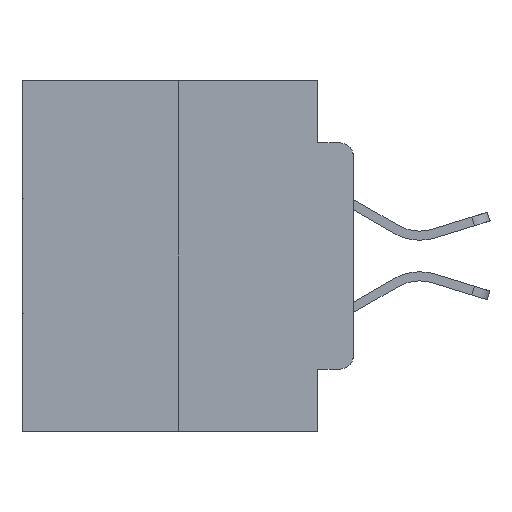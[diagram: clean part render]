
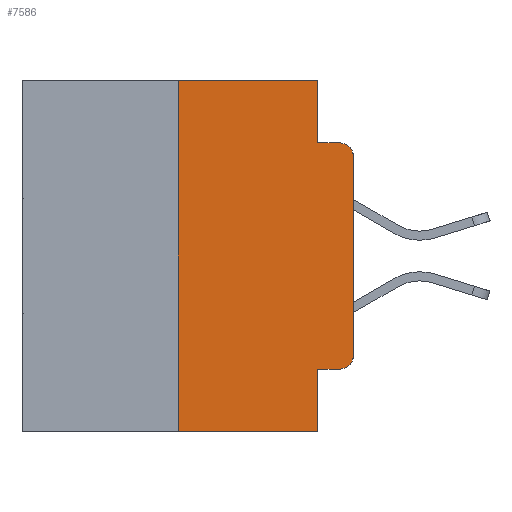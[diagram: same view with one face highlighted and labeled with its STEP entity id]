
A CAD part, left-side view. The second image highlights one B-rep face of the part: STEP entity #7586.
In plain terms, the highlighted planar face has unit normal (-1, 0, 0).
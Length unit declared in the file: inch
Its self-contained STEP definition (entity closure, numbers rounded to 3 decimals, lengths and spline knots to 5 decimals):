
#863 = ORIENTED_EDGE ( 'NONE', *, *, #16979, .F. ) ;
#1055 = CARTESIAN_POINT ( 'NONE',  ( 0., 0.25, -0.5 ) ) ;
#2234 = CIRCLE ( 'NONE', #12386, 0.02 ) ;
#2438 = ORIENTED_EDGE ( 'NONE', *, *, #23348, .F. ) ;
#4496 = CARTESIAN_POINT ( 'NONE',  ( 0., 0.051, 0. ) ) ;
#4684 = CARTESIAN_POINT ( 'NONE',  ( 0., 0., 0. ) ) ;
#5418 = VERTEX_POINT ( 'NONE', #18519 ) ;
#5578 = DIRECTION ( 'NONE',  ( 0., 0., -1. ) ) ;
#5652 = VECTOR ( 'NONE', #28266, 39.37008 ) ;
#5811 = VERTEX_POINT ( 'NONE', #4496 ) ;
#6142 = PLANE ( 'NONE',  #23346 ) ;
#6863 = LINE ( 'NONE', #19147, #18099 ) ;
#7013 = DIRECTION ( 'NONE',  ( 0., 0., 1. ) ) ;
#7075 = VECTOR ( 'NONE', #21052, 39.37008 ) ;
#7295 = LINE ( 'NONE', #7904, #19167 ) ;
#7436 = VERTEX_POINT ( 'NONE', #27648 ) ;
#7541 = LINE ( 'NONE', #4684, #18737 ) ;
#7586 = ADVANCED_FACE ( 'NONE', ( #21837 ), #6142, .F. ) ;
#7904 = CARTESIAN_POINT ( 'NONE',  ( 0., 0.051, 0. ) ) ;
#8372 = EDGE_CURVE ( 'NONE', #18516, #13982, #7541, .T. ) ;
#8602 = LINE ( 'NONE', #24713, #13903 ) ;
#8946 = CARTESIAN_POINT ( 'NONE',  ( 0., 0.051, -0.0885 ) ) ;
#9190 = EDGE_CURVE ( 'NONE', #9930, #7436, #15619, .T. ) ;
#9440 = ORIENTED_EDGE ( 'NONE', *, *, #9190, .F. ) ;
#9930 = VERTEX_POINT ( 'NONE', #1055 ) ;
#10231 = CARTESIAN_POINT ( 'NONE',  ( 0., 0.02, -0.1085 ) ) ;
#10759 = DIRECTION ( 'NONE',  ( 1., 0., 0. ) ) ;
#10763 = CARTESIAN_POINT ( 'NONE',  ( 0., 0.051, -0.0885 ) ) ;
#10794 = DIRECTION ( 'NONE',  ( -1., 0., 0. ) ) ;
#11306 = EDGE_CURVE ( 'NONE', #18978, #19253, #11762, .T. ) ;
#11553 = LINE ( 'NONE', #10763, #15380 ) ;
#11762 = LINE ( 'NONE', #23798, #5652 ) ;
#12197 = CIRCLE ( 'NONE', #22020, 0.02 ) ;
#12225 = VERTEX_POINT ( 'NONE', #18252 ) ;
#12356 = CARTESIAN_POINT ( 'NONE',  ( 0., 0.25, 0. ) ) ;
#12386 = AXIS2_PLACEMENT_3D ( 'NONE', #23962, #10794, #26143 ) ;
#12526 = DIRECTION ( 'NONE',  ( 0., 0., -1. ) ) ;
#12571 = CARTESIAN_POINT ( 'NONE',  ( 0., 0., -0.3915 ) ) ;
#13034 = DIRECTION ( 'NONE',  ( 0., -1., 0. ) ) ;
#13781 = CARTESIAN_POINT ( 'NONE',  ( 0., 0.02, -0.4115 ) ) ;
#13903 = VECTOR ( 'NONE', #26909, 39.37008 ) ;
#13982 = VERTEX_POINT ( 'NONE', #26884 ) ;
#14579 = DIRECTION ( 'NONE',  ( 0., 0., 1. ) ) ;
#14798 = ORIENTED_EDGE ( 'NONE', *, *, #15962, .T. ) ;
#14876 = EDGE_CURVE ( 'NONE', #18978, #12225, #7295, .T. ) ;
#15380 = VECTOR ( 'NONE', #13034, 39.37008 ) ;
#15619 = LINE ( 'NONE', #12356, #26497 ) ;
#15663 = EDGE_CURVE ( 'NONE', #23685, #5418, #11553, .T. ) ;
#15962 = EDGE_CURVE ( 'NONE', #9930, #12225, #6863, .T. ) ;
#16979 = EDGE_CURVE ( 'NONE', #5811, #23685, #8602, .T. ) ;
#17646 = ORIENTED_EDGE ( 'NONE', *, *, #8372, .T. ) ;
#18099 = VECTOR ( 'NONE', #27902, 39.37008 ) ;
#18252 = CARTESIAN_POINT ( 'NONE',  ( 0., 0.051, -0.5 ) ) ;
#18516 = VERTEX_POINT ( 'NONE', #12571 ) ;
#18519 = CARTESIAN_POINT ( 'NONE',  ( 0., 0.02, -0.0885 ) ) ;
#18580 = EDGE_LOOP ( 'NONE', ( #17646, #19224, #22054, #863, #2438, #9440, #14798, #27046, #25819, #27656 ) ) ;
#18631 = EDGE_CURVE ( 'NONE', #19253, #18516, #2234, .T. ) ;
#18737 = VECTOR ( 'NONE', #7013, 39.37008 ) ;
#18978 = VERTEX_POINT ( 'NONE', #19439 ) ;
#19147 = CARTESIAN_POINT ( 'NONE',  ( 0., 0.473, -0.5 ) ) ;
#19167 = VECTOR ( 'NONE', #5578, 39.37008 ) ;
#19224 = ORIENTED_EDGE ( 'NONE', *, *, #24616, .T. ) ;
#19253 = VERTEX_POINT ( 'NONE', #13781 ) ;
#19439 = CARTESIAN_POINT ( 'NONE',  ( 0., 0.051, -0.4115 ) ) ;
#21052 = DIRECTION ( 'NONE',  ( 0., -1., 0. ) ) ;
#21726 = CARTESIAN_POINT ( 'NONE',  ( 0., 0.473, 0. ) ) ;
#21837 = FACE_OUTER_BOUND ( 'NONE', #18580, .T. ) ;
#22020 = AXIS2_PLACEMENT_3D ( 'NONE', #10231, #25628, #12526 ) ;
#22054 = ORIENTED_EDGE ( 'NONE', *, *, #15663, .F. ) ;
#23346 = AXIS2_PLACEMENT_3D ( 'NONE', #21726, #10759, #26107 ) ;
#23348 = EDGE_CURVE ( 'NONE', #7436, #5811, #24760, .T. ) ;
#23685 = VERTEX_POINT ( 'NONE', #8946 ) ;
#23798 = CARTESIAN_POINT ( 'NONE',  ( 0., 0.051, -0.4115 ) ) ;
#23962 = CARTESIAN_POINT ( 'NONE',  ( 0., 0.02, -0.3915 ) ) ;
#24616 = EDGE_CURVE ( 'NONE', #13982, #5418, #12197, .T. ) ;
#24713 = CARTESIAN_POINT ( 'NONE',  ( 0., 0.051, 0. ) ) ;
#24760 = LINE ( 'NONE', #27640, #7075 ) ;
#25628 = DIRECTION ( 'NONE',  ( -1., 0., 0. ) ) ;
#25819 = ORIENTED_EDGE ( 'NONE', *, *, #11306, .T. ) ;
#26107 = DIRECTION ( 'NONE',  ( 0., 0., -1. ) ) ;
#26143 = DIRECTION ( 'NONE',  ( 0., 0., -1. ) ) ;
#26497 = VECTOR ( 'NONE', #14579, 39.37008 ) ;
#26884 = CARTESIAN_POINT ( 'NONE',  ( 0., 0., -0.1085 ) ) ;
#26909 = DIRECTION ( 'NONE',  ( 0., 0., -1. ) ) ;
#27046 = ORIENTED_EDGE ( 'NONE', *, *, #14876, .F. ) ;
#27640 = CARTESIAN_POINT ( 'NONE',  ( 0., 0.473, 0. ) ) ;
#27648 = CARTESIAN_POINT ( 'NONE',  ( 0., 0.25, 0. ) ) ;
#27656 = ORIENTED_EDGE ( 'NONE', *, *, #18631, .T. ) ;
#27902 = DIRECTION ( 'NONE',  ( 0., -1., 0. ) ) ;
#28266 = DIRECTION ( 'NONE',  ( 0., -1., 0. ) ) ;
